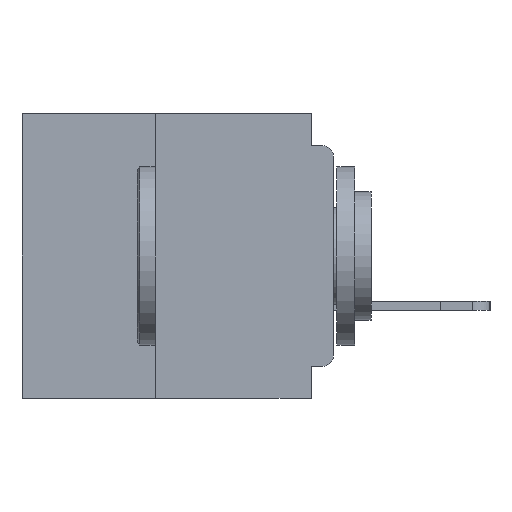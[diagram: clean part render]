
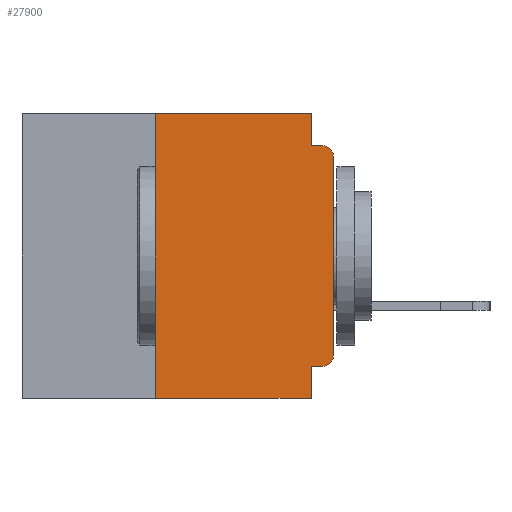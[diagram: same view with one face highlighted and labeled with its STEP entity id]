
A CAD part, left-side view. The second image highlights one B-rep face of the part: STEP entity #27900.
In plain terms, the highlighted planar face has unit normal (-1, 0, 0).
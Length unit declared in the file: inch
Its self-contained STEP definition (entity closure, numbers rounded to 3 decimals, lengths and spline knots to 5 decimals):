
#265 = ORIENTED_EDGE ( 'NONE', *, *, #30393, .F. ) ;
#929 = VERTEX_POINT ( 'NONE', #18472 ) ;
#1114 = CARTESIAN_POINT ( 'NONE',  ( 0., 0.25, -0.4 ) ) ;
#1346 = CARTESIAN_POINT ( 'NONE',  ( 0., 0., -0.06 ) ) ;
#1370 = CARTESIAN_POINT ( 'NONE',  ( 0., 0.031, -0.045 ) ) ;
#1510 = CARTESIAN_POINT ( 'NONE',  ( 0., 0.031, -0.355 ) ) ;
#2181 = CARTESIAN_POINT ( 'NONE',  ( 0., 0.25, -0.4 ) ) ;
#2344 = EDGE_CURVE ( 'NONE', #39646, #929, #32896, .T. ) ;
#3000 = CARTESIAN_POINT ( 'NONE',  ( 0., 0., 0. ) ) ;
#3401 = EDGE_CURVE ( 'NONE', #4212, #33325, #11099, .T. ) ;
#3487 = PLANE ( 'NONE',  #31199 ) ;
#3723 = DIRECTION ( 'NONE',  ( 0., -1., 0. ) ) ;
#4056 = LINE ( 'NONE', #2181, #36694 ) ;
#4194 = VERTEX_POINT ( 'NONE', #33874 ) ;
#4212 = VERTEX_POINT ( 'NONE', #33236 ) ;
#4941 = DIRECTION ( 'NONE',  ( 0., 1., 0. ) ) ;
#5230 = ORIENTED_EDGE ( 'NONE', *, *, #34782, .F. ) ;
#5909 = EDGE_CURVE ( 'NONE', #929, #36450, #21144, .T. ) ;
#6790 = DIRECTION ( 'NONE',  ( 0., 0., -1. ) ) ;
#6825 = EDGE_LOOP ( 'NONE', ( #13451, #40674, #32941, #13144, #16906, #5230, #22966, #265, #16861, #38613 ) ) ;
#7782 = LINE ( 'NONE', #33620, #14337 ) ;
#7932 = FACE_OUTER_BOUND ( 'NONE', #6825, .T. ) ;
#8982 = DIRECTION ( 'NONE',  ( -1., 0., 0. ) ) ;
#10119 = CARTESIAN_POINT ( 'NONE',  ( 0., 0., -0.045 ) ) ;
#11016 = EDGE_CURVE ( 'NONE', #36450, #25622, #39987, .T. ) ;
#11099 = LINE ( 'NONE', #28888, #35112 ) ;
#11751 = VECTOR ( 'NONE', #36020, 39.37008 ) ;
#12785 = LINE ( 'NONE', #31492, #29086 ) ;
#13144 = ORIENTED_EDGE ( 'NONE', *, *, #3401, .F. ) ;
#13308 = EDGE_CURVE ( 'NONE', #4194, #4212, #20402, .T. ) ;
#13451 = ORIENTED_EDGE ( 'NONE', *, *, #5909, .T. ) ;
#14337 = VECTOR ( 'NONE', #23872, 39.37008 ) ;
#15694 = VECTOR ( 'NONE', #3723, 39.37008 ) ;
#16861 = ORIENTED_EDGE ( 'NONE', *, *, #19766, .F. ) ;
#16906 = ORIENTED_EDGE ( 'NONE', *, *, #13308, .F. ) ;
#17913 = CARTESIAN_POINT ( 'NONE',  ( 0., 0.015, -0.355 ) ) ;
#18472 = CARTESIAN_POINT ( 'NONE',  ( 0., 0., -0.34 ) ) ;
#19766 = EDGE_CURVE ( 'NONE', #39646, #25809, #28929, .T. ) ;
#19873 = CARTESIAN_POINT ( 'NONE',  ( 0., 0.015, -0.045 ) ) ;
#20262 = VECTOR ( 'NONE', #4941, 39.37008 ) ;
#20402 = LINE ( 'NONE', #22860, #11751 ) ;
#21144 = LINE ( 'NONE', #3000, #29833 ) ;
#22860 = CARTESIAN_POINT ( 'NONE',  ( 0., 0.437, 0. ) ) ;
#22925 = DIRECTION ( 'NONE',  ( 0., 0., -1. ) ) ;
#22935 = CARTESIAN_POINT ( 'NONE',  ( 0., 0.437, 0. ) ) ;
#22966 = ORIENTED_EDGE ( 'NONE', *, *, #32596, .T. ) ;
#22972 = DIRECTION ( 'NONE',  ( -1., 0., 0. ) ) ;
#23119 = CARTESIAN_POINT ( 'NONE',  ( 0., 0.015, -0.34 ) ) ;
#23872 = DIRECTION ( 'NONE',  ( 0., -1., 0. ) ) ;
#24351 = LINE ( 'NONE', #10119, #15694 ) ;
#25622 = VERTEX_POINT ( 'NONE', #19873 ) ;
#25809 = VERTEX_POINT ( 'NONE', #1510 ) ;
#26218 = DIRECTION ( 'NONE',  ( 1., 0., 0. ) ) ;
#26545 = AXIS2_PLACEMENT_3D ( 'NONE', #28479, #8982, #31782 ) ;
#27900 = ADVANCED_FACE ( 'NONE', ( #7932 ), #3487, .F. ) ;
#28197 = DIRECTION ( 'NONE',  ( 0., 0., -1. ) ) ;
#28479 = CARTESIAN_POINT ( 'NONE',  ( 0., 0.015, -0.06 ) ) ;
#28888 = CARTESIAN_POINT ( 'NONE',  ( 0., 0.031, 0. ) ) ;
#28929 = LINE ( 'NONE', #34152, #20262 ) ;
#29086 = VECTOR ( 'NONE', #28197, 39.37008 ) ;
#29324 = DIRECTION ( 'NONE',  ( 0., 0., -1. ) ) ;
#29833 = VECTOR ( 'NONE', #38746, 39.37008 ) ;
#30393 = EDGE_CURVE ( 'NONE', #25809, #37667, #12785, .T. ) ;
#31199 = AXIS2_PLACEMENT_3D ( 'NONE', #22935, #26218, #6790 ) ;
#31275 = AXIS2_PLACEMENT_3D ( 'NONE', #23119, #22972, #22925 ) ;
#31492 = CARTESIAN_POINT ( 'NONE',  ( 0., 0.031, -0.4 ) ) ;
#31782 = DIRECTION ( 'NONE',  ( 0., 0., -1. ) ) ;
#32596 = EDGE_CURVE ( 'NONE', #35793, #37667, #7782, .T. ) ;
#32896 = CIRCLE ( 'NONE', #31275, 0.015 ) ;
#32941 = ORIENTED_EDGE ( 'NONE', *, *, #35100, .F. ) ;
#33236 = CARTESIAN_POINT ( 'NONE',  ( 0., 0.031, 0. ) ) ;
#33325 = VERTEX_POINT ( 'NONE', #1370 ) ;
#33620 = CARTESIAN_POINT ( 'NONE',  ( 0., 0.437, -0.4 ) ) ;
#33874 = CARTESIAN_POINT ( 'NONE',  ( 0., 0.25, 0. ) ) ;
#34152 = CARTESIAN_POINT ( 'NONE',  ( 0., 0., -0.355 ) ) ;
#34782 = EDGE_CURVE ( 'NONE', #35793, #4194, #4056, .T. ) ;
#35100 = EDGE_CURVE ( 'NONE', #33325, #25622, #24351, .T. ) ;
#35112 = VECTOR ( 'NONE', #29324, 39.37008 ) ;
#35793 = VERTEX_POINT ( 'NONE', #1114 ) ;
#36020 = DIRECTION ( 'NONE',  ( 0., -1., 0. ) ) ;
#36450 = VERTEX_POINT ( 'NONE', #1346 ) ;
#36694 = VECTOR ( 'NONE', #41169, 39.37008 ) ;
#37201 = CARTESIAN_POINT ( 'NONE',  ( 0., 0.031, -0.4 ) ) ;
#37667 = VERTEX_POINT ( 'NONE', #37201 ) ;
#38613 = ORIENTED_EDGE ( 'NONE', *, *, #2344, .T. ) ;
#38746 = DIRECTION ( 'NONE',  ( 0., 0., 1. ) ) ;
#39646 = VERTEX_POINT ( 'NONE', #17913 ) ;
#39987 = CIRCLE ( 'NONE', #26545, 0.015 ) ;
#40674 = ORIENTED_EDGE ( 'NONE', *, *, #11016, .T. ) ;
#41169 = DIRECTION ( 'NONE',  ( 0., 0., 1. ) ) ;
